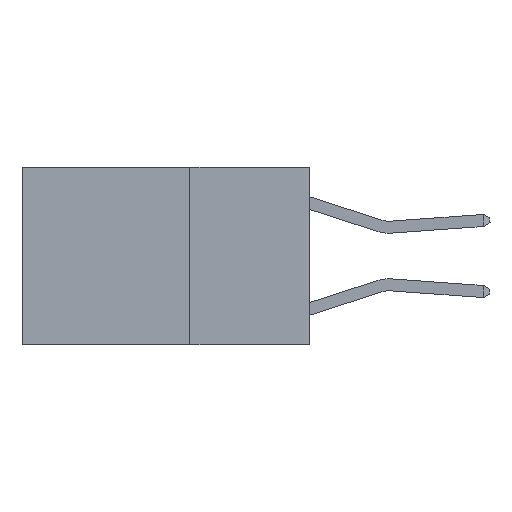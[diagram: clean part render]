
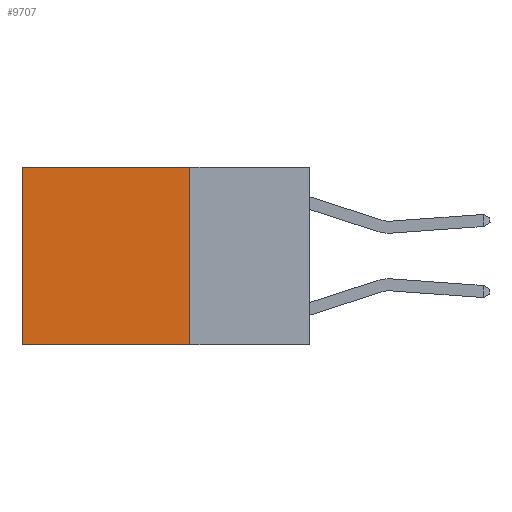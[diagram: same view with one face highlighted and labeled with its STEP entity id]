
A CAD part, left-side view. The second image highlights one B-rep face of the part: STEP entity #9707.
In plain terms, the highlighted planar face has unit normal (-1, 0, 0).
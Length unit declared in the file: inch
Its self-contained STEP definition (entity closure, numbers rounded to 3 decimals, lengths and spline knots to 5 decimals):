
#601 = LINE ( 'NONE', #12924, #6116 ) ;
#1350 = ORIENTED_EDGE ( 'NONE', *, *, #5575, .F. ) ;
#1681 = CARTESIAN_POINT ( 'NONE',  ( 0.2625, 0.25, 0. ) ) ;
#1724 = CARTESIAN_POINT ( 'NONE',  ( 0.2625, 0.25, 0. ) ) ;
#3071 = FACE_OUTER_BOUND ( 'NONE', #8428, .T. ) ;
#3119 = LINE ( 'NONE', #12013, #8560 ) ;
#3606 = EDGE_CURVE ( 'NONE', #12738, #5939, #4475, .T. ) ;
#3882 = CARTESIAN_POINT ( 'NONE',  ( 0.2625, 0.6, -0.37 ) ) ;
#4323 = DIRECTION ( 'NONE',  ( 0., 1., 0. ) ) ;
#4475 = LINE ( 'NONE', #13421, #12033 ) ;
#5575 = EDGE_CURVE ( 'NONE', #12738, #11328, #601, .T. ) ;
#5578 = EDGE_CURVE ( 'NONE', #5939, #6768, #3119, .T. ) ;
#5581 = CARTESIAN_POINT ( 'NONE',  ( 0.2625, 0.25, -0.37 ) ) ;
#5590 = CARTESIAN_POINT ( 'NONE',  ( 0.2625, 0.6, 0. ) ) ;
#5939 = VERTEX_POINT ( 'NONE', #5590 ) ;
#6116 = VECTOR ( 'NONE', #10982, 39.37008 ) ;
#6193 = PLANE ( 'NONE',  #12730 ) ;
#6657 = EDGE_CURVE ( 'NONE', #11328, #6768, #6952, .T. ) ;
#6768 = VERTEX_POINT ( 'NONE', #3882 ) ;
#6952 = LINE ( 'NONE', #9053, #9351 ) ;
#7288 = DIRECTION ( 'NONE',  ( 0., 0., -1. ) ) ;
#8428 = EDGE_LOOP ( 'NONE', ( #12792, #9879, #1350, #8654 ) ) ;
#8560 = VECTOR ( 'NONE', #12963, 39.37008 ) ;
#8654 = ORIENTED_EDGE ( 'NONE', *, *, #3606, .T. ) ;
#9053 = CARTESIAN_POINT ( 'NONE',  ( 0.2625, 0.25, -0.37 ) ) ;
#9351 = VECTOR ( 'NONE', #10041, 39.37008 ) ;
#9707 = ADVANCED_FACE ( 'NONE', ( #3071 ), #6193, .F. ) ;
#9879 = ORIENTED_EDGE ( 'NONE', *, *, #6657, .F. ) ;
#10041 = DIRECTION ( 'NONE',  ( 0., 1., 0. ) ) ;
#10982 = DIRECTION ( 'NONE',  ( 0., 0., -1. ) ) ;
#11328 = VERTEX_POINT ( 'NONE', #5581 ) ;
#12013 = CARTESIAN_POINT ( 'NONE',  ( 0.2625, 0.6, 0. ) ) ;
#12033 = VECTOR ( 'NONE', #4323, 39.37008 ) ;
#12730 = AXIS2_PLACEMENT_3D ( 'NONE', #1724, #13176, #7288 ) ;
#12738 = VERTEX_POINT ( 'NONE', #1681 ) ;
#12792 = ORIENTED_EDGE ( 'NONE', *, *, #5578, .T. ) ;
#12924 = CARTESIAN_POINT ( 'NONE',  ( 0.2625, 0.25, 0. ) ) ;
#12963 = DIRECTION ( 'NONE',  ( 0., 0., -1. ) ) ;
#13176 = DIRECTION ( 'NONE',  ( 1., 0., 0. ) ) ;
#13421 = CARTESIAN_POINT ( 'NONE',  ( 0.2625, 0.25, 0. ) ) ;
